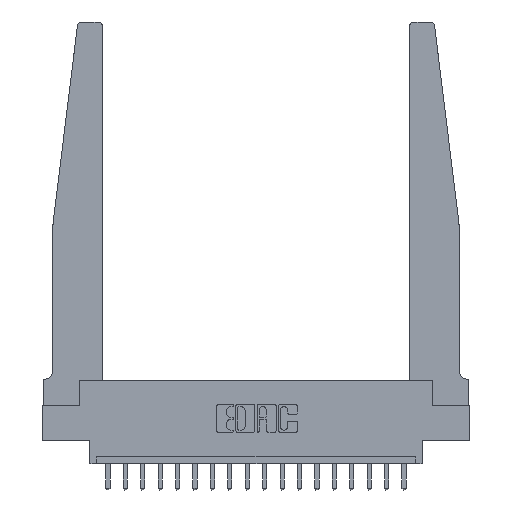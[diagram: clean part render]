
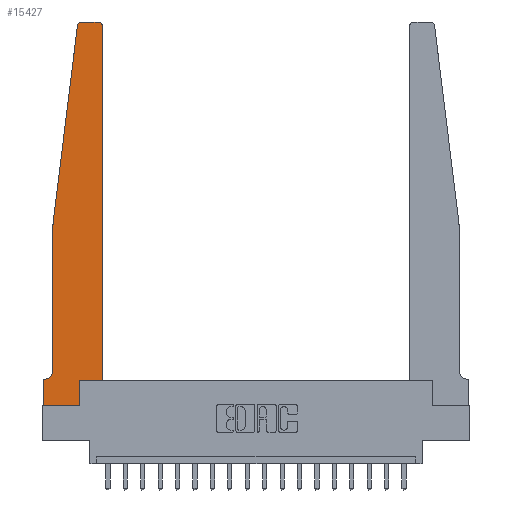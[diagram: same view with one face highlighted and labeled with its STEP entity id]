
A CAD part, top view. The second image highlights one B-rep face of the part: STEP entity #15427.
In plain terms, the highlighted planar face has unit normal (0, 0, 1).
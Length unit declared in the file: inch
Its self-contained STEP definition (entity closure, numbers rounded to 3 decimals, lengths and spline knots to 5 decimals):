
#9 = LINE ( 'NONE', #19208, #7769 ) ;
#181 = DIRECTION ( 'NONE',  ( 1., 0., 0. ) ) ;
#492 = VECTOR ( 'NONE', #7542, 39.37008 ) ;
#529 = EDGE_CURVE ( 'NONE', #4843, #18179, #7770, .T. ) ;
#1001 = EDGE_CURVE ( 'NONE', #6124, #4843, #10561, .T. ) ;
#1039 = VECTOR ( 'NONE', #6848, 39.37008 ) ;
#1130 = ORIENTED_EDGE ( 'NONE', *, *, #1001, .T. ) ;
#1507 = ORIENTED_EDGE ( 'NONE', *, *, #15016, .T. ) ;
#2287 = CARTESIAN_POINT ( 'NONE',  ( 0.2605, 0., 0.37 ) ) ;
#2323 = ORIENTED_EDGE ( 'NONE', *, *, #13346, .T. ) ;
#2386 = CARTESIAN_POINT ( 'NONE',  ( 0.015, 0.2375, 0.37 ) ) ;
#2676 = VECTOR ( 'NONE', #7469, 39.37008 ) ;
#2702 = LINE ( 'NONE', #4120, #1039 ) ;
#2713 = CARTESIAN_POINT ( 'NONE',  ( 0.24675, 2.72367, 0.37 ) ) ;
#2906 = ORIENTED_EDGE ( 'NONE', *, *, #10770, .T. ) ;
#2922 = DIRECTION ( 'NONE',  ( 1., 0., 0. ) ) ;
#3134 = ORIENTED_EDGE ( 'NONE', *, *, #12585, .T. ) ;
#3475 = VERTEX_POINT ( 'NONE', #8302 ) ;
#3568 = CARTESIAN_POINT ( 'NONE',  ( 0., 0.1875, 0.37 ) ) ;
#3694 = CARTESIAN_POINT ( 'NONE',  ( 0.425, 0.18, 0.37 ) ) ;
#3870 = DIRECTION ( 'NONE',  ( 1., 0., 0. ) ) ;
#3901 = DIRECTION ( 'NONE',  ( 0., 0., -1. ) ) ;
#3923 = VERTEX_POINT ( 'NONE', #16043 ) ;
#3978 = ORIENTED_EDGE ( 'NONE', *, *, #529, .T. ) ;
#4051 = LINE ( 'NONE', #8733, #7532 ) ;
#4120 = CARTESIAN_POINT ( 'NONE',  ( 0., 0., 0.37 ) ) ;
#4843 = VERTEX_POINT ( 'NONE', #8175 ) ;
#4913 = VERTEX_POINT ( 'NONE', #9379 ) ;
#5000 = CARTESIAN_POINT ( 'NONE',  ( 0.395, 2.72, 0.37 ) ) ;
#5331 = CIRCLE ( 'NONE', #10604, 0.05 ) ;
#5492 = CARTESIAN_POINT ( 'NONE',  ( 0.065, 0.1875, 0.37 ) ) ;
#6124 = VERTEX_POINT ( 'NONE', #11968 ) ;
#6268 = VERTEX_POINT ( 'NONE', #2287 ) ;
#6376 = EDGE_CURVE ( 'NONE', #8541, #4913, #17309, .T. ) ;
#6510 = DIRECTION ( 'NONE',  ( 0., -1., 0. ) ) ;
#6578 = VERTEX_POINT ( 'NONE', #15321 ) ;
#6617 = AXIS2_PLACEMENT_3D ( 'NONE', #5000, #9176, #181 ) ;
#6848 = DIRECTION ( 'NONE',  ( 0., -1., 0. ) ) ;
#6922 = CARTESIAN_POINT ( 'NONE',  ( 0.27653, 2.72, 0.37 ) ) ;
#7464 = VERTEX_POINT ( 'NONE', #15909 ) ;
#7469 = DIRECTION ( 'NONE',  ( 0., 1., 0. ) ) ;
#7532 = VECTOR ( 'NONE', #13295, 39.37008 ) ;
#7542 = DIRECTION ( 'NONE',  ( -1., 0., 0. ) ) ;
#7579 = AXIS2_PLACEMENT_3D ( 'NONE', #6922, #8371, #3870 ) ;
#7769 = VECTOR ( 'NONE', #2922, 39.37008 ) ;
#7770 = CIRCLE ( 'NONE', #6617, 0.03 ) ;
#8001 = DIRECTION ( 'NONE',  ( -0.122, -0.992, 0. ) ) ;
#8175 = CARTESIAN_POINT ( 'NONE',  ( 0.425, 2.72, 0.37 ) ) ;
#8194 = EDGE_CURVE ( 'NONE', #6268, #10225, #9241, .T. ) ;
#8216 = PLANE ( 'NONE',  #12784 ) ;
#8302 = CARTESIAN_POINT ( 'NONE',  ( 0.27653, 2.75, 0.37 ) ) ;
#8371 = DIRECTION ( 'NONE',  ( 0., 0., 1. ) ) ;
#8541 = VERTEX_POINT ( 'NONE', #17253 ) ;
#8733 = CARTESIAN_POINT ( 'NONE',  ( 0.425, 0.18, 0.37 ) ) ;
#9176 = DIRECTION ( 'NONE',  ( 0., 0., 1. ) ) ;
#9191 = EDGE_CURVE ( 'NONE', #18179, #3475, #15098, .T. ) ;
#9241 = LINE ( 'NONE', #16430, #2676 ) ;
#9331 = ORIENTED_EDGE ( 'NONE', *, *, #9191, .T. ) ;
#9343 = CARTESIAN_POINT ( 'NONE',  ( 0.395, 2.75, 0.37 ) ) ;
#9379 = CARTESIAN_POINT ( 'NONE',  ( 0.065, 0.2375, 0.37 ) ) ;
#9382 = ORIENTED_EDGE ( 'NONE', *, *, #8194, .T. ) ;
#9601 = ORIENTED_EDGE ( 'NONE', *, *, #13024, .T. ) ;
#9794 = EDGE_CURVE ( 'NONE', #10225, #6124, #4051, .T. ) ;
#10157 = VECTOR ( 'NONE', #14448, 39.37008 ) ;
#10225 = VERTEX_POINT ( 'NONE', #17178 ) ;
#10561 = LINE ( 'NONE', #3694, #14362 ) ;
#10604 = AXIS2_PLACEMENT_3D ( 'NONE', #2386, #3901, #14416 ) ;
#10770 = EDGE_CURVE ( 'NONE', #7464, #6268, #9, .T. ) ;
#10997 = CARTESIAN_POINT ( 'NONE',  ( 0.065, 1.25, 0.37 ) ) ;
#11131 = DIRECTION ( 'NONE',  ( 1., 0., 0. ) ) ;
#11968 = CARTESIAN_POINT ( 'NONE',  ( 0.425, 0.18, 0.37 ) ) ;
#12585 = EDGE_CURVE ( 'NONE', #15220, #8541, #18014, .T. ) ;
#12602 = VECTOR ( 'NONE', #6510, 39.37008 ) ;
#12784 = AXIS2_PLACEMENT_3D ( 'NONE', #3568, #15799, #11131 ) ;
#12799 = EDGE_LOOP ( 'NONE', ( #9331, #9601, #3134, #19370, #2323, #1507, #18238, #2906, #9382, #15489, #1130, #3978 ) ) ;
#13024 = EDGE_CURVE ( 'NONE', #3475, #15220, #13331, .T. ) ;
#13295 = DIRECTION ( 'NONE',  ( 1., 0., 0. ) ) ;
#13331 = CIRCLE ( 'NONE', #7579, 0.03 ) ;
#13346 = EDGE_CURVE ( 'NONE', #4913, #6578, #5331, .T. ) ;
#13463 = CARTESIAN_POINT ( 'NONE',  ( 0.25, 2.75, 0.37 ) ) ;
#14362 = VECTOR ( 'NONE', #16281, 39.37008 ) ;
#14416 = DIRECTION ( 'NONE',  ( -1., 0., 0. ) ) ;
#14448 = DIRECTION ( 'NONE',  ( -1., 0., 0. ) ) ;
#15016 = EDGE_CURVE ( 'NONE', #6578, #3923, #17920, .T. ) ;
#15098 = LINE ( 'NONE', #13463, #492 ) ;
#15220 = VERTEX_POINT ( 'NONE', #2713 ) ;
#15321 = CARTESIAN_POINT ( 'NONE',  ( 0.015, 0.1875, 0.37 ) ) ;
#15427 = ADVANCED_FACE ( 'NONE', ( #15595 ), #8216, .T. ) ;
#15489 = ORIENTED_EDGE ( 'NONE', *, *, #9794, .T. ) ;
#15524 = CARTESIAN_POINT ( 'NONE',  ( 0.065, 1.25, 0.37 ) ) ;
#15595 = FACE_OUTER_BOUND ( 'NONE', #12799, .T. ) ;
#15799 = DIRECTION ( 'NONE',  ( 0., 0., 1. ) ) ;
#15909 = CARTESIAN_POINT ( 'NONE',  ( 0., 0., 0.37 ) ) ;
#16043 = CARTESIAN_POINT ( 'NONE',  ( 0., 0.1875, 0.37 ) ) ;
#16163 = VECTOR ( 'NONE', #8001, 39.37008 ) ;
#16281 = DIRECTION ( 'NONE',  ( 0., 1., 0. ) ) ;
#16430 = CARTESIAN_POINT ( 'NONE',  ( 0.2605, 0.18, 0.37 ) ) ;
#17178 = CARTESIAN_POINT ( 'NONE',  ( 0.2605, 0.18, 0.37 ) ) ;
#17253 = CARTESIAN_POINT ( 'NONE',  ( 0.065, 1.25, 0.37 ) ) ;
#17309 = LINE ( 'NONE', #15524, #12602 ) ;
#17400 = EDGE_CURVE ( 'NONE', #3923, #7464, #2702, .T. ) ;
#17920 = LINE ( 'NONE', #5492, #10157 ) ;
#18014 = LINE ( 'NONE', #10997, #16163 ) ;
#18179 = VERTEX_POINT ( 'NONE', #9343 ) ;
#18238 = ORIENTED_EDGE ( 'NONE', *, *, #17400, .T. ) ;
#19208 = CARTESIAN_POINT ( 'NONE',  ( 0., 0., 0.37 ) ) ;
#19370 = ORIENTED_EDGE ( 'NONE', *, *, #6376, .T. ) ;
